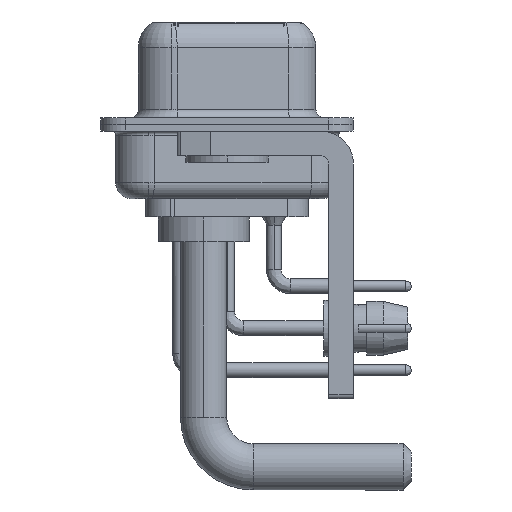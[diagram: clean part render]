
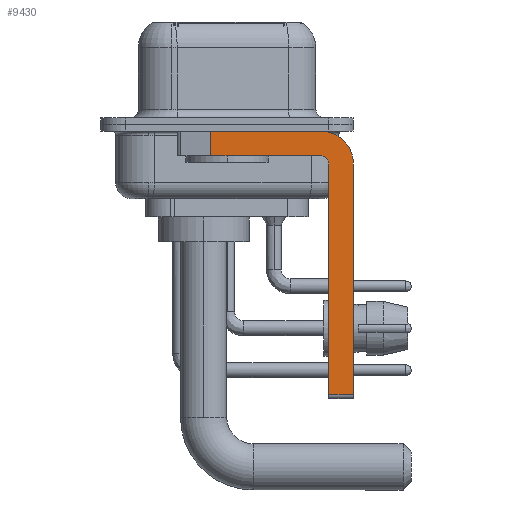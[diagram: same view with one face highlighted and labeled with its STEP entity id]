
A CAD part, left-side view. The second image highlights one B-rep face of the part: STEP entity #9430.
In plain terms, the highlighted planar face has unit normal (-1, 0, 0).
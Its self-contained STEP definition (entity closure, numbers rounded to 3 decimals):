
#516 = ORIENTED_EDGE ( 'NONE', *, *, #12489, .F. ) ;
#898 = EDGE_CURVE ( 'NONE', #12331, #12160, #6588, .T. ) ;
#1480 = ORIENTED_EDGE ( 'NONE', *, *, #8347, .F. ) ;
#2259 = CARTESIAN_POINT ( 'NONE',  ( -2.9, -5.65, -16.35 ) ) ;
#2470 = CARTESIAN_POINT ( 'NONE',  ( -2.9, -7.65, -2.4 ) ) ;
#2647 = VERTEX_POINT ( 'NONE', #11166 ) ;
#2943 = CARTESIAN_POINT ( 'NONE',  ( -2.9, -5.65, -1.9 ) ) ;
#3727 = DIRECTION ( 'NONE',  ( 0., 0., -1. ) ) ;
#5200 = LINE ( 'NONE', #2470, #28106 ) ;
#5461 = AXIS2_PLACEMENT_3D ( 'NONE', #29572, #29391, #6937 ) ;
#5929 = CARTESIAN_POINT ( 'NONE',  ( -2.9, -5.65, -2.4 ) ) ;
#6588 = CIRCLE ( 'NONE', #22445, 0.5 ) ;
#6937 = DIRECTION ( 'NONE',  ( 0., 0., -1. ) ) ;
#8347 = EDGE_CURVE ( 'NONE', #14785, #35875, #5200, .T. ) ;
#9430 = ADVANCED_FACE ( 'NONE', ( #28561 ), #31705, .F. ) ;
#10068 = LINE ( 'NONE', #32542, #27297 ) ;
#10855 = LINE ( 'NONE', #2259, #14495 ) ;
#11166 = CARTESIAN_POINT ( 'NONE',  ( -2.9, -5.65, -0.4 ) ) ;
#11231 = CARTESIAN_POINT ( 'NONE',  ( -2.9, -7.65, -16.35 ) ) ;
#11849 = VERTEX_POINT ( 'NONE', #19279 ) ;
#12160 = VERTEX_POINT ( 'NONE', #2943 ) ;
#12331 = VERTEX_POINT ( 'NONE', #29029 ) ;
#12489 = EDGE_CURVE ( 'NONE', #2647, #14785, #24837, .T. ) ;
#13186 = CARTESIAN_POINT ( 'NONE',  ( -2.9, 3., -0.4 ) ) ;
#13255 = VECTOR ( 'NONE', #24404, 1000. ) ;
#14033 = VECTOR ( 'NONE', #14251, 1000. ) ;
#14251 = DIRECTION ( 'NONE',  ( 0., 0., 1. ) ) ;
#14495 = VECTOR ( 'NONE', #22062, 1000. ) ;
#14785 = VERTEX_POINT ( 'NONE', #32584 ) ;
#15078 = ORIENTED_EDGE ( 'NONE', *, *, #17467, .T. ) ;
#15203 = DIRECTION ( 'NONE',  ( 0., 0., -1. ) ) ;
#16082 = VECTOR ( 'NONE', #20760, 1000. ) ;
#17282 = CARTESIAN_POINT ( 'NONE',  ( -2.9, -5.65, -1.9 ) ) ;
#17463 = LINE ( 'NONE', #17282, #16082 ) ;
#17467 = EDGE_CURVE ( 'NONE', #11849, #35875, #10855, .T. ) ;
#18732 = ORIENTED_EDGE ( 'NONE', *, *, #898, .F. ) ;
#19098 = DIRECTION ( 'NONE',  ( -1., 0., 0. ) ) ;
#19279 = CARTESIAN_POINT ( 'NONE',  ( -2.9, -6.15, -16.35 ) ) ;
#19585 = CARTESIAN_POINT ( 'NONE',  ( -2.9, -6.15, -16.6 ) ) ;
#19927 = VERTEX_POINT ( 'NONE', #28821 ) ;
#20760 = DIRECTION ( 'NONE',  ( 0., 1., 0. ) ) ;
#22062 = DIRECTION ( 'NONE',  ( 0., -1., 0. ) ) ;
#22445 = AXIS2_PLACEMENT_3D ( 'NONE', #28325, #19098, #27590 ) ;
#22715 = LINE ( 'NONE', #19585, #14033 ) ;
#22915 = EDGE_CURVE ( 'NONE', #11849, #12331, #22715, .T. ) ;
#23530 = AXIS2_PLACEMENT_3D ( 'NONE', #5929, #28740, #3727 ) ;
#24404 = DIRECTION ( 'NONE',  ( 0., -1., 0. ) ) ;
#24837 = CIRCLE ( 'NONE', #5461, 2. ) ;
#27188 = LINE ( 'NONE', #13186, #13255 ) ;
#27297 = VECTOR ( 'NONE', #15203, 1000. ) ;
#27590 = DIRECTION ( 'NONE',  ( 0., 0., 1. ) ) ;
#28106 = VECTOR ( 'NONE', #32334, 1000. ) ;
#28325 = CARTESIAN_POINT ( 'NONE',  ( -2.9, -5.65, -2.4 ) ) ;
#28561 = FACE_OUTER_BOUND ( 'NONE', #30941, .T. ) ;
#28740 = DIRECTION ( 'NONE',  ( 1., 0., 0. ) ) ;
#28821 = CARTESIAN_POINT ( 'NONE',  ( -2.9, 0.978, -0.4 ) ) ;
#29029 = CARTESIAN_POINT ( 'NONE',  ( -2.9, -6.15, -2.4 ) ) ;
#29391 = DIRECTION ( 'NONE',  ( 1., 0., 0. ) ) ;
#29572 = CARTESIAN_POINT ( 'NONE',  ( -2.9, -5.65, -2.4 ) ) ;
#30067 = CARTESIAN_POINT ( 'NONE',  ( -2.9, 0.978, -1.9 ) ) ;
#30448 = EDGE_CURVE ( 'NONE', #12160, #35234, #17463, .T. ) ;
#30744 = ORIENTED_EDGE ( 'NONE', *, *, #31064, .T. ) ;
#30941 = EDGE_LOOP ( 'NONE', ( #36118, #30744, #33260, #18732, #31345, #15078, #1480, #516 ) ) ;
#31064 = EDGE_CURVE ( 'NONE', #19927, #35234, #10068, .T. ) ;
#31345 = ORIENTED_EDGE ( 'NONE', *, *, #22915, .F. ) ;
#31705 = PLANE ( 'NONE',  #23530 ) ;
#32334 = DIRECTION ( 'NONE',  ( 0., 0., -1. ) ) ;
#32500 = EDGE_CURVE ( 'NONE', #19927, #2647, #27188, .T. ) ;
#32542 = CARTESIAN_POINT ( 'NONE',  ( -2.9, 0.978, -1.9 ) ) ;
#32584 = CARTESIAN_POINT ( 'NONE',  ( -2.9, -7.65, -2.4 ) ) ;
#33260 = ORIENTED_EDGE ( 'NONE', *, *, #30448, .F. ) ;
#35234 = VERTEX_POINT ( 'NONE', #30067 ) ;
#35875 = VERTEX_POINT ( 'NONE', #11231 ) ;
#36118 = ORIENTED_EDGE ( 'NONE', *, *, #32500, .F. ) ;
